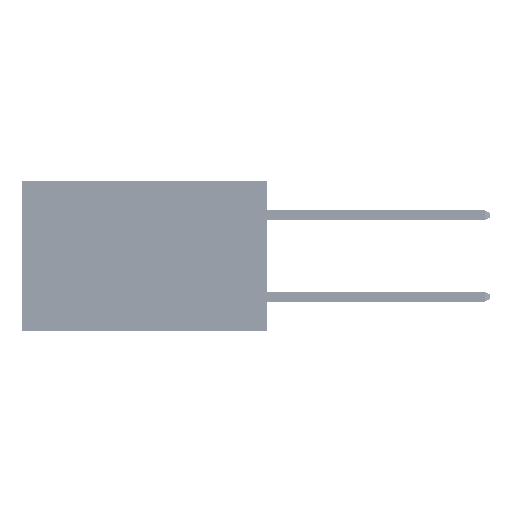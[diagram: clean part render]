
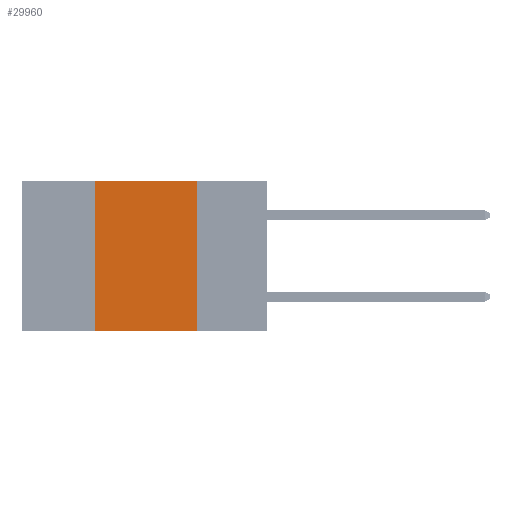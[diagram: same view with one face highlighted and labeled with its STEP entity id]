
A CAD part, left-side view. The second image highlights one B-rep face of the part: STEP entity #29960.
In plain terms, the highlighted planar face has unit normal (-1, 0, 0).
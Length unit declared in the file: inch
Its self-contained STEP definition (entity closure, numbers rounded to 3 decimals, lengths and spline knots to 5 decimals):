
#74 = CARTESIAN_POINT ( 'NONE',  ( 0., 0.17, 0. ) ) ;
#7807 = VECTOR ( 'NONE', #17105, 39.37008 ) ;
#9278 = CARTESIAN_POINT ( 'NONE',  ( 0., 0.6, 0. ) ) ;
#9672 = CARTESIAN_POINT ( 'NONE',  ( 0., 0.6, 0. ) ) ;
#12076 = AXIS2_PLACEMENT_3D ( 'NONE', #9672, #32691, #17145 ) ;
#13038 = ORIENTED_EDGE ( 'NONE', *, *, #21613, .F. ) ;
#15067 = ORIENTED_EDGE ( 'NONE', *, *, #45183, .T. ) ;
#15662 = VERTEX_POINT ( 'NONE', #46850 ) ;
#17007 = EDGE_CURVE ( 'NONE', #15662, #24119, #30379, .T. ) ;
#17105 = DIRECTION ( 'NONE',  ( 0., -1., 0. ) ) ;
#17145 = DIRECTION ( 'NONE',  ( 0., 0., -1. ) ) ;
#19386 = ORIENTED_EDGE ( 'NONE', *, *, #17007, .F. ) ;
#21613 = EDGE_CURVE ( 'NONE', #23147, #26132, #28107, .T. ) ;
#22213 = DIRECTION ( 'NONE',  ( 0., 0., 1. ) ) ;
#22972 = LINE ( 'NONE', #27020, #50229 ) ;
#23147 = VERTEX_POINT ( 'NONE', #74 ) ;
#24119 = VERTEX_POINT ( 'NONE', #37559 ) ;
#24588 = EDGE_LOOP ( 'NONE', ( #13038, #43126, #19386, #15067 ) ) ;
#24646 = DIRECTION ( 'NONE',  ( 0., 0., -1. ) ) ;
#25156 = LINE ( 'NONE', #9278, #7807 ) ;
#26132 = VERTEX_POINT ( 'NONE', #26649 ) ;
#26649 = CARTESIAN_POINT ( 'NONE',  ( 0., 0.17, -0.37 ) ) ;
#27020 = CARTESIAN_POINT ( 'NONE',  ( 0., 0.6, -0.37 ) ) ;
#28107 = LINE ( 'NONE', #41085, #44195 ) ;
#29734 = VECTOR ( 'NONE', #22213, 39.37008 ) ;
#29960 = ADVANCED_FACE ( 'NONE', ( #42040 ), #48619, .F. ) ;
#30379 = LINE ( 'NONE', #49383, #29734 ) ;
#32691 = DIRECTION ( 'NONE',  ( 1., 0., 0. ) ) ;
#34989 = DIRECTION ( 'NONE',  ( 0., -1., 0. ) ) ;
#35480 = EDGE_CURVE ( 'NONE', #24119, #23147, #25156, .T. ) ;
#37559 = CARTESIAN_POINT ( 'NONE',  ( 0., 0.42, 0. ) ) ;
#41085 = CARTESIAN_POINT ( 'NONE',  ( 0., 0.17, 0. ) ) ;
#42040 = FACE_OUTER_BOUND ( 'NONE', #24588, .T. ) ;
#43126 = ORIENTED_EDGE ( 'NONE', *, *, #35480, .F. ) ;
#44195 = VECTOR ( 'NONE', #24646, 39.37008 ) ;
#45183 = EDGE_CURVE ( 'NONE', #15662, #26132, #22972, .T. ) ;
#46850 = CARTESIAN_POINT ( 'NONE',  ( 0., 0.42, -0.37 ) ) ;
#48619 = PLANE ( 'NONE',  #12076 ) ;
#49383 = CARTESIAN_POINT ( 'NONE',  ( 0., 0.42, 0. ) ) ;
#50229 = VECTOR ( 'NONE', #34989, 39.37008 ) ;
